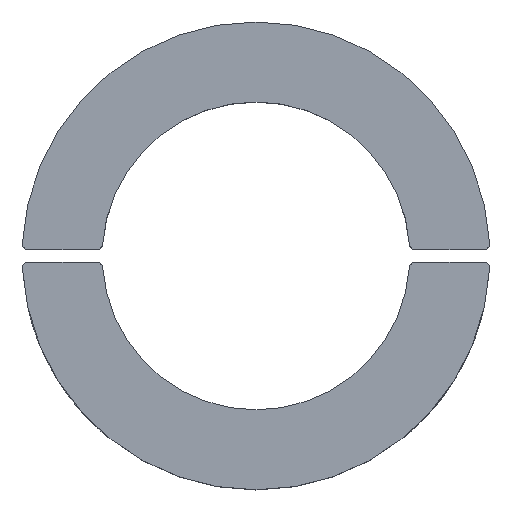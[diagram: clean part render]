
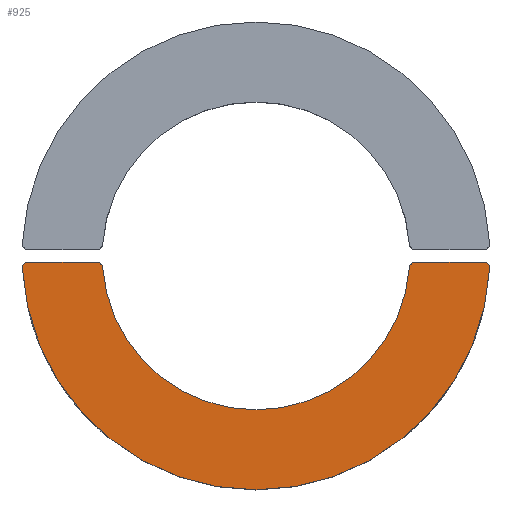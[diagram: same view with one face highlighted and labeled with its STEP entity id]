
A CAD part, top view. The second image highlights one B-rep face of the part: STEP entity #925.
In plain terms, the highlighted planar face has unit normal (0, 0, 1).
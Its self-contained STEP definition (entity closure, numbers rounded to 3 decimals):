
#60=PLANE('',#1039);
#137=FACE_OUTER_BOUND('',#207,.T.);
#207=EDGE_LOOP('',(#827,#828,#829,#830,#831,#832,#833,#834));
#252=LINE('',#2286,#314);
#258=LINE('',#2303,#320);
#314=VECTOR('',#1243,10.);
#320=VECTOR('',#1259,10.);
#364=CIRCLE('',#992,19.);
#384=CIRCLE('',#1035,0.5);
#385=CIRCLE('',#1037,0.5);
#386=CIRCLE('',#1040,12.5);
#387=CIRCLE('',#1041,0.5);
#388=CIRCLE('',#1042,0.5);
#429=VERTEX_POINT('',#1862);
#430=VERTEX_POINT('',#1864);
#443=VERTEX_POINT('',#2283);
#444=VERTEX_POINT('',#2285);
#449=VERTEX_POINT('',#2300);
#450=VERTEX_POINT('',#2302);
#461=VERTEX_POINT('',#2349);
#462=VERTEX_POINT('',#2354);
#531=EDGE_CURVE('',#430,#429,#364,.T.);
#552=EDGE_CURVE('',#444,#443,#252,.T.);
#560=EDGE_CURVE('',#450,#449,#258,.T.);
#584=EDGE_CURVE('',#444,#429,#384,.T.);
#586=EDGE_CURVE('',#461,#443,#385,.T.);
#587=EDGE_CURVE('',#461,#462,#386,.T.);
#588=EDGE_CURVE('',#450,#462,#387,.T.);
#589=EDGE_CURVE('',#430,#449,#388,.T.);
#827=ORIENTED_EDGE('',*,*,#586,.F.);
#828=ORIENTED_EDGE('',*,*,#587,.T.);
#829=ORIENTED_EDGE('',*,*,#588,.F.);
#830=ORIENTED_EDGE('',*,*,#560,.T.);
#831=ORIENTED_EDGE('',*,*,#589,.F.);
#832=ORIENTED_EDGE('',*,*,#531,.T.);
#833=ORIENTED_EDGE('',*,*,#584,.F.);
#834=ORIENTED_EDGE('',*,*,#552,.T.);
#925=ADVANCED_FACE('',(#137),#60,.T.);
#992=AXIS2_PLACEMENT_3D('',#1865,#1201,#1202);
#1035=AXIS2_PLACEMENT_3D('',#2347,#1314,#1315);
#1037=AXIS2_PLACEMENT_3D('',#2351,#1319,#1320);
#1039=AXIS2_PLACEMENT_3D('',#2353,#1323,#1324);
#1040=AXIS2_PLACEMENT_3D('',#2355,#1325,#1326);
#1041=AXIS2_PLACEMENT_3D('',#2356,#1327,#1328);
#1042=AXIS2_PLACEMENT_3D('',#2357,#1329,#1330);
#1201=DIRECTION('center_axis',(0.,0.,1.));
#1202=DIRECTION('ref_axis',(1.,0.,0.));
#1243=DIRECTION('',(-1.,0.,0.));
#1259=DIRECTION('',(-1.,0.,0.));
#1314=DIRECTION('center_axis',(0.,0.,-1.));
#1315=DIRECTION('ref_axis',(0.726,0.688,0.));
#1319=DIRECTION('center_axis',(0.,0.,-1.));
#1320=DIRECTION('ref_axis',(-0.679,0.734,0.));
#1323=DIRECTION('center_axis',(0.,0.,1.));
#1324=DIRECTION('ref_axis',(1.,0.,0.));
#1325=DIRECTION('center_axis',(0.,0.,-1.));
#1326=DIRECTION('ref_axis',(1.,0.,0.));
#1327=DIRECTION('center_axis',(0.,0.,-1.));
#1328=DIRECTION('ref_axis',(0.679,0.734,0.));
#1329=DIRECTION('center_axis',(0.,0.,-1.));
#1330=DIRECTION('ref_axis',(-0.726,0.688,0.));
#1862=CARTESIAN_POINT('',(18.972,-1.027,8.));
#1864=CARTESIAN_POINT('',(-18.972,-1.027,8.));
#1865=CARTESIAN_POINT('Origin',(0.,0.,8.));
#2283=CARTESIAN_POINT('',(12.961,-0.5,8.));
#2285=CARTESIAN_POINT('',(18.473,-0.5,8.));
#2286=CARTESIAN_POINT('',(18.993,-0.5,8.));
#2300=CARTESIAN_POINT('',(-18.473,-0.5,8.));
#2302=CARTESIAN_POINT('',(-12.961,-0.5,8.));
#2303=CARTESIAN_POINT('',(18.993,-0.5,8.));
#2347=CARTESIAN_POINT('Origin',(18.473,-1.,8.));
#2349=CARTESIAN_POINT('',(12.463,-0.962,8.));
#2351=CARTESIAN_POINT('Origin',(12.961,-1.,8.));
#2353=CARTESIAN_POINT('Origin',(0.,-9.75,
8.));
#2354=CARTESIAN_POINT('',(-12.463,-0.962,8.));
#2355=CARTESIAN_POINT('Origin',(0.,0.,8.));
#2356=CARTESIAN_POINT('Origin',(-12.961,-1.,8.));
#2357=CARTESIAN_POINT('Origin',(-18.473,-1.,8.));
